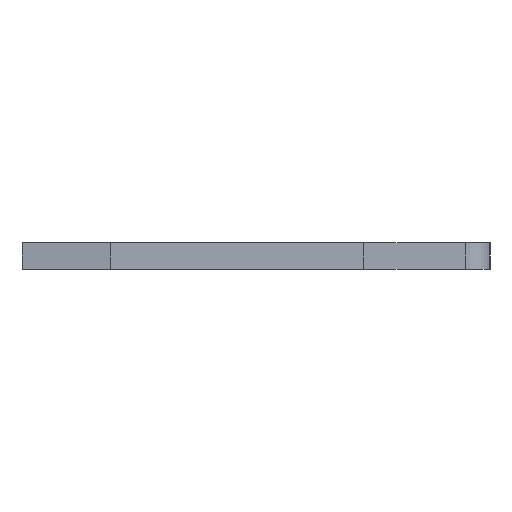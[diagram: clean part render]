
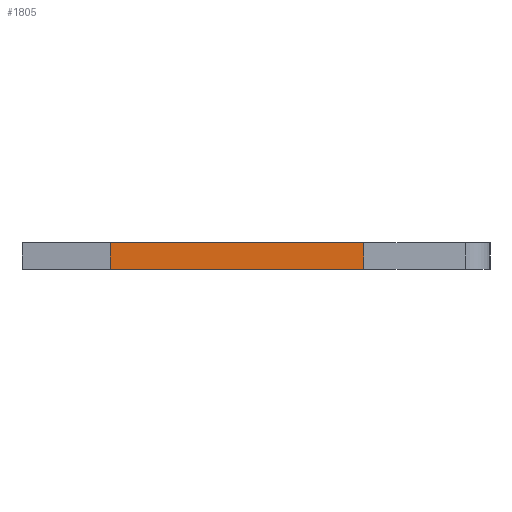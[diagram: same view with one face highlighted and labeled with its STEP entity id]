
A CAD part, left-side view. The second image highlights one B-rep face of the part: STEP entity #1805.
In plain terms, the highlighted face is planar.
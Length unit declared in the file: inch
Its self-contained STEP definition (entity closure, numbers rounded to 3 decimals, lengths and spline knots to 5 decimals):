
#20 = ORIENTED_EDGE ( 'NONE', *, *, #1949, .T. ) ;
#32 = VERTEX_POINT ( 'NONE', #1009 ) ;
#45 = CARTESIAN_POINT ( 'NONE',  ( 0.013, 0.146, -0.0575 ) ) ;
#51 = FACE_OUTER_BOUND ( 'NONE', #1517, .T. ) ;
#100 = LINE ( 'NONE', #1028, #1723 ) ;
#167 = ORIENTED_EDGE ( 'NONE', *, *, #1296, .T. ) ;
#208 = ORIENTED_EDGE ( 'NONE', *, *, #1134, .F. ) ;
#259 = DIRECTION ( 'NONE',  ( -1., 0., 0. ) ) ;
#506 = CARTESIAN_POINT ( 'NONE',  ( 0.013, 0.146, -0.0575 ) ) ;
#545 = VECTOR ( 'NONE', #1479, 39.37008 ) ;
#624 = AXIS2_PLACEMENT_3D ( 'NONE', #1364, #1208, #1537 ) ;
#672 = DIRECTION ( 'NONE',  ( 0., 1., 0. ) ) ;
#836 = CARTESIAN_POINT ( 'NONE',  ( -0.013, -0.099, -0.0575 ) ) ;
#868 = EDGE_CURVE ( 'NONE', #1289, #1345, #100, .T. ) ;
#874 = LINE ( 'NONE', #1643, #1714 ) ;
#898 = PLANE ( 'NONE',  #624 ) ;
#919 = ORIENTED_EDGE ( 'NONE', *, *, #868, .F. ) ;
#1009 = CARTESIAN_POINT ( 'NONE',  ( -0.013, 0.146, -0.0575 ) ) ;
#1028 = CARTESIAN_POINT ( 'NONE',  ( 0.013, 0.146, -0.0575 ) ) ;
#1134 = EDGE_CURVE ( 'NONE', #1345, #32, #1977, .T. ) ;
#1160 = CARTESIAN_POINT ( 'NONE',  ( 0.013, -0.099, -0.0575 ) ) ;
#1208 = DIRECTION ( 'NONE',  ( 0., 0., 1. ) ) ;
#1289 = VERTEX_POINT ( 'NONE', #1160 ) ;
#1290 = VERTEX_POINT ( 'NONE', #836 ) ;
#1296 = EDGE_CURVE ( 'NONE', #1290, #32, #874, .T. ) ;
#1345 = VERTEX_POINT ( 'NONE', #506 ) ;
#1364 = CARTESIAN_POINT ( 'NONE',  ( 0.013, 0.146, -0.0575 ) ) ;
#1424 = DIRECTION ( 'NONE',  ( 0., 1., 0. ) ) ;
#1479 = DIRECTION ( 'NONE',  ( -1., 0., 0. ) ) ;
#1517 = EDGE_LOOP ( 'NONE', ( #167, #208, #919, #20 ) ) ;
#1537 = DIRECTION ( 'NONE',  ( 1., 0., 0. ) ) ;
#1543 = VECTOR ( 'NONE', #259, 39.37008 ) ;
#1643 = CARTESIAN_POINT ( 'NONE',  ( -0.013, 0.146, -0.0575 ) ) ;
#1714 = VECTOR ( 'NONE', #672, 39.37008 ) ;
#1723 = VECTOR ( 'NONE', #1424, 39.37008 ) ;
#1805 = ADVANCED_FACE ( 'NONE', ( #51 ), #898, .F. ) ;
#1949 = EDGE_CURVE ( 'NONE', #1289, #1290, #1987, .T. ) ;
#1977 = LINE ( 'NONE', #45, #545 ) ;
#1987 = LINE ( 'NONE', #2026, #1543 ) ;
#2026 = CARTESIAN_POINT ( 'NONE',  ( 0.013, -0.099, -0.0575 ) ) ;
